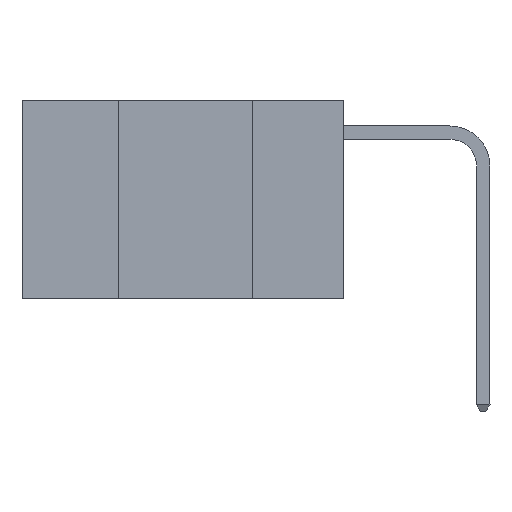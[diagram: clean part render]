
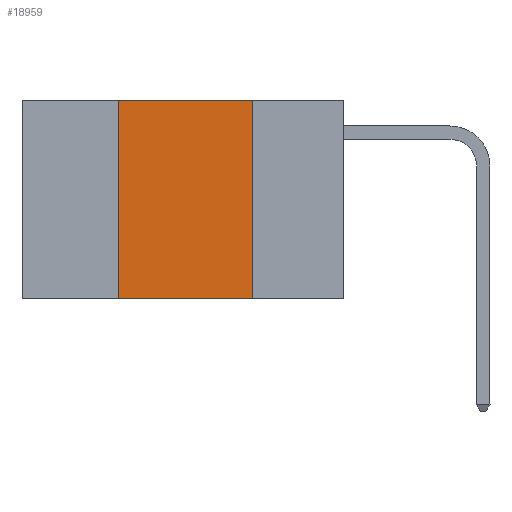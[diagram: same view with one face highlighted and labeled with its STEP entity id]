
A CAD part, left-side view. The second image highlights one B-rep face of the part: STEP entity #18959.
In plain terms, the highlighted planar face has unit normal (-1, 0, 0).
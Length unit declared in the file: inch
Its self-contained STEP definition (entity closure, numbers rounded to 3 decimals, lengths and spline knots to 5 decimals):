
#1680 = LINE ( 'NONE', #22335, #20673 ) ;
#1894 = CARTESIAN_POINT ( 'NONE',  ( 0., 0.42, 0. ) ) ;
#2315 = LINE ( 'NONE', #11914, #20917 ) ;
#2670 = DIRECTION ( 'NONE',  ( 0., 0., -1. ) ) ;
#2742 = CARTESIAN_POINT ( 'NONE',  ( 0., 0.17, 0. ) ) ;
#3568 = CARTESIAN_POINT ( 'NONE',  ( 0., 0.42, 0. ) ) ;
#3764 = VERTEX_POINT ( 'NONE', #3568 ) ;
#4478 = DIRECTION ( 'NONE',  ( 0., 0., 1. ) ) ;
#5095 = EDGE_LOOP ( 'NONE', ( #22887, #15682, #8860, #20641 ) ) ;
#5929 = VERTEX_POINT ( 'NONE', #21384 ) ;
#6225 = VERTEX_POINT ( 'NONE', #16524 ) ;
#6345 = EDGE_CURVE ( 'NONE', #3764, #20967, #1680, .T. ) ;
#8860 = ORIENTED_EDGE ( 'NONE', *, *, #12886, .F. ) ;
#9280 = DIRECTION ( 'NONE',  ( 0., -1., 0. ) ) ;
#10989 = EDGE_CURVE ( 'NONE', #6225, #5929, #16625, .T. ) ;
#11914 = CARTESIAN_POINT ( 'NONE',  ( 0., 0.17, 0. ) ) ;
#12186 = DIRECTION ( 'NONE',  ( 1., 0., 0. ) ) ;
#12441 = VECTOR ( 'NONE', #4478, 39.37008 ) ;
#12515 = CARTESIAN_POINT ( 'NONE',  ( 0., 0.6, -0.37 ) ) ;
#12772 = DIRECTION ( 'NONE',  ( 0., -1., 0. ) ) ;
#12886 = EDGE_CURVE ( 'NONE', #6225, #3764, #13834, .T. ) ;
#13834 = LINE ( 'NONE', #1894, #12441 ) ;
#13960 = FACE_OUTER_BOUND ( 'NONE', #5095, .T. ) ;
#15682 = ORIENTED_EDGE ( 'NONE', *, *, #6345, .F. ) ;
#15957 = DIRECTION ( 'NONE',  ( 0., 0., -1. ) ) ;
#16524 = CARTESIAN_POINT ( 'NONE',  ( 0., 0.42, -0.37 ) ) ;
#16625 = LINE ( 'NONE', #12515, #20093 ) ;
#17044 = AXIS2_PLACEMENT_3D ( 'NONE', #23588, #12186, #15957 ) ;
#18959 = ADVANCED_FACE ( 'NONE', ( #13960 ), #21507, .F. ) ;
#19983 = EDGE_CURVE ( 'NONE', #20967, #5929, #2315, .T. ) ;
#20093 = VECTOR ( 'NONE', #12772, 39.37008 ) ;
#20641 = ORIENTED_EDGE ( 'NONE', *, *, #10989, .T. ) ;
#20673 = VECTOR ( 'NONE', #9280, 39.37008 ) ;
#20917 = VECTOR ( 'NONE', #2670, 39.37008 ) ;
#20967 = VERTEX_POINT ( 'NONE', #2742 ) ;
#21384 = CARTESIAN_POINT ( 'NONE',  ( 0., 0.17, -0.37 ) ) ;
#21507 = PLANE ( 'NONE',  #17044 ) ;
#22335 = CARTESIAN_POINT ( 'NONE',  ( 0., 0.6, 0. ) ) ;
#22887 = ORIENTED_EDGE ( 'NONE', *, *, #19983, .F. ) ;
#23588 = CARTESIAN_POINT ( 'NONE',  ( 0., 0.6, 0. ) ) ;
